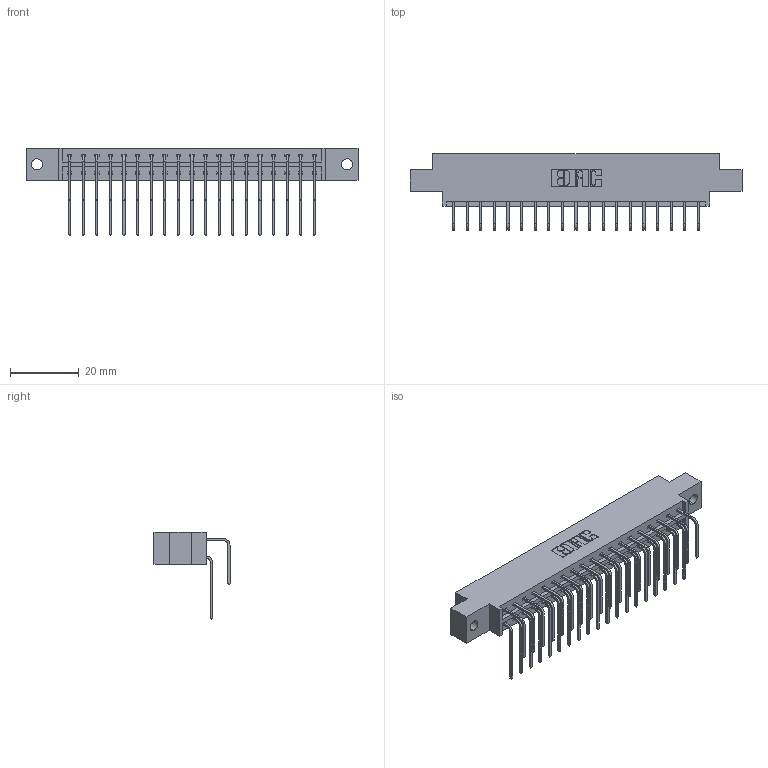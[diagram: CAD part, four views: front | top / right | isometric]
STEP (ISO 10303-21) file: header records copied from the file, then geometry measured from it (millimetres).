
FILE_DESCRIPTION (( 'STEP AP203' ), '1' );
FILE_NAME ('333-038-558-802.STEP', '2018-08-03T12:06:51', ( '' ), ( '' ), 'SwSTEP 2.0', 'SolidWorks 2016', '' );
FILE_SCHEMA (( 'CONFIG_CONTROL_DESIGN' ));
Length unit declared in the file: inch
Products named in the file (4): 333 Part_Offset - .128 Dia; 345-292-001_558 559 Tail - 1; 345-292-001_558 Tail - 2; 333-038-558-802
Assembly tree (39 placements, depth 2):
  333-038-558-802
    333 Part_Offset - .128 Dia
    345-292-001_558 559 Tail - 1  x19
    345-292-001_558 Tail - 2  x19
Bounding box: 96.82 x 22.17 x 25.53 mm (x, y, z)
Volume: 9624.9 mm3; surface area: 12171.3 mm2
Topology: 39 solids, 39 shells, 2170 faces, 6441 edges, 4242 vertices
Faces by surface type: plane 1518, cylinder 652
Entity records: 17117 total; most frequent: CARTESIAN_POINT 2917, ORIENTED_EDGE 2802, DIRECTION 2513, EDGE_CURVE 1401, VECTOR 1233, LINE 1233, VERTEX_POINT 930, AXIS2_PLACEMENT_3D 640
